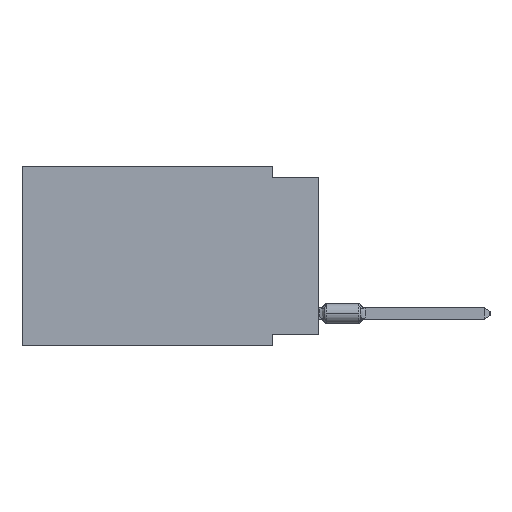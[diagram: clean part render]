
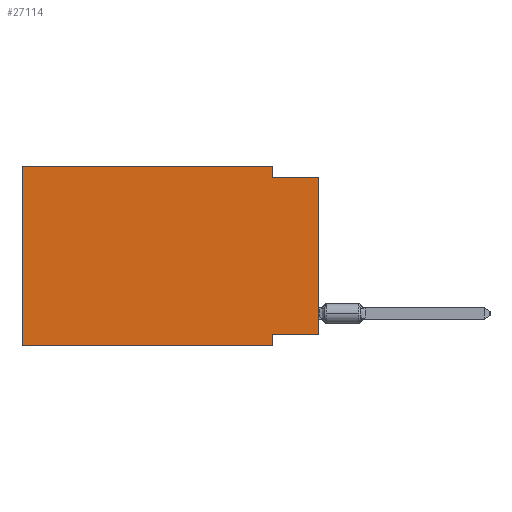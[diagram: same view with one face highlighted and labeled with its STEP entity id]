
A CAD part, left-side view. The second image highlights one B-rep face of the part: STEP entity #27114.
In plain terms, the highlighted planar face has unit normal (-1, 0, 0).
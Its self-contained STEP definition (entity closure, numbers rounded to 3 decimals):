
#895 = DIRECTION ( 'NONE',  ( 0., 0., 1. ) ) ;
#1077 = DIRECTION ( 'NONE',  ( 0., 1., 0. ) ) ;
#1387 = DIRECTION ( 'NONE',  ( 0., 0., -1. ) ) ;
#2608 = VECTOR ( 'NONE', #9329, 1000. ) ;
#2900 = EDGE_CURVE ( 'NONE', #19758, #13571, #29375, .T. ) ;
#4257 = VERTEX_POINT ( 'NONE', #18093 ) ;
#5572 = CARTESIAN_POINT ( 'NONE',  ( 0., 2.54, -9.906 ) ) ;
#6136 = FACE_OUTER_BOUND ( 'NONE', #12895, .T. ) ;
#7039 = EDGE_CURVE ( 'NONE', #14759, #13571, #8423, .T. ) ;
#7259 = ORIENTED_EDGE ( 'NONE', *, *, #7039, .F. ) ;
#8343 = ORIENTED_EDGE ( 'NONE', *, *, #2900, .T. ) ;
#8423 = LINE ( 'NONE', #20137, #11509 ) ;
#8878 = ORIENTED_EDGE ( 'NONE', *, *, #21564, .F. ) ;
#9329 = DIRECTION ( 'NONE',  ( 0., 0., -1. ) ) ;
#9922 = VECTOR ( 'NONE', #16440, 1000. ) ;
#10450 = VECTOR ( 'NONE', #895, 1000. ) ;
#11478 = VERTEX_POINT ( 'NONE', #32034 ) ;
#11509 = VECTOR ( 'NONE', #33464, 1000. ) ;
#12895 = EDGE_LOOP ( 'NONE', ( #8343, #7259, #27799, #15864, #33020, #26986, #20630, #8878 ) ) ;
#13352 = VERTEX_POINT ( 'NONE', #29213 ) ;
#13571 = VERTEX_POINT ( 'NONE', #32173 ) ;
#14233 = LINE ( 'NONE', #27930, #25042 ) ;
#14759 = VERTEX_POINT ( 'NONE', #18105 ) ;
#14871 = LINE ( 'NONE', #30676, #16644 ) ;
#15864 = ORIENTED_EDGE ( 'NONE', *, *, #25416, .F. ) ;
#16440 = DIRECTION ( 'NONE',  ( 0., -1., 0. ) ) ;
#16511 = VECTOR ( 'NONE', #20960, 1000. ) ;
#16644 = VECTOR ( 'NONE', #28745, 1000. ) ;
#18093 = CARTESIAN_POINT ( 'NONE',  ( 0., 16.383, -9.906 ) ) ;
#18105 = CARTESIAN_POINT ( 'NONE',  ( 0., 2.54, -0.635 ) ) ;
#18322 = CARTESIAN_POINT ( 'NONE',  ( 0., 0., 0. ) ) ;
#18431 = VECTOR ( 'NONE', #31993, 1000. ) ;
#19678 = LINE ( 'NONE', #33195, #2608 ) ;
#19758 = VERTEX_POINT ( 'NONE', #32919 ) ;
#20137 = CARTESIAN_POINT ( 'NONE',  ( 0., 0., -0.635 ) ) ;
#20284 = EDGE_CURVE ( 'NONE', #13352, #29763, #14871, .T. ) ;
#20630 = ORIENTED_EDGE ( 'NONE', *, *, #20284, .F. ) ;
#20960 = DIRECTION ( 'NONE',  ( 0., 0., 1. ) ) ;
#21283 = LINE ( 'NONE', #21970, #18431 ) ;
#21564 = EDGE_CURVE ( 'NONE', #19758, #13352, #14233, .T. ) ;
#21599 = EDGE_CURVE ( 'NONE', #27079, #14759, #19678, .T. ) ;
#21616 = EDGE_CURVE ( 'NONE', #4257, #11478, #27582, .T. ) ;
#21970 = CARTESIAN_POINT ( 'NONE',  ( 0., 16.383, 0. ) ) ;
#25042 = VECTOR ( 'NONE', #1077, 1000. ) ;
#25416 = EDGE_CURVE ( 'NONE', #11478, #27079, #21283, .T. ) ;
#26986 = ORIENTED_EDGE ( 'NONE', *, *, #27311, .T. ) ;
#27079 = VERTEX_POINT ( 'NONE', #30191 ) ;
#27114 = ADVANCED_FACE ( 'NONE', ( #6136 ), #30903, .F. ) ;
#27311 = EDGE_CURVE ( 'NONE', #4257, #29763, #34710, .T. ) ;
#27582 = LINE ( 'NONE', #27745, #10450 ) ;
#27745 = CARTESIAN_POINT ( 'NONE',  ( 0., 16.383, 0. ) ) ;
#27799 = ORIENTED_EDGE ( 'NONE', *, *, #21599, .F. ) ;
#27930 = CARTESIAN_POINT ( 'NONE',  ( 0., 0., -9.271 ) ) ;
#28075 = CARTESIAN_POINT ( 'NONE',  ( 0., 16.383, 0. ) ) ;
#28745 = DIRECTION ( 'NONE',  ( 0., 0., -1. ) ) ;
#29213 = CARTESIAN_POINT ( 'NONE',  ( 0., 2.54, -9.271 ) ) ;
#29375 = LINE ( 'NONE', #18322, #16511 ) ;
#29763 = VERTEX_POINT ( 'NONE', #5572 ) ;
#29797 = CARTESIAN_POINT ( 'NONE',  ( 0., 16.383, -9.906 ) ) ;
#30191 = CARTESIAN_POINT ( 'NONE',  ( 0., 2.54, 0. ) ) ;
#30676 = CARTESIAN_POINT ( 'NONE',  ( 0., 2.54, -9.906 ) ) ;
#30903 = PLANE ( 'NONE',  #31989 ) ;
#31989 = AXIS2_PLACEMENT_3D ( 'NONE', #28075, #32811, #1387 ) ;
#31993 = DIRECTION ( 'NONE',  ( 0., -1., 0. ) ) ;
#32034 = CARTESIAN_POINT ( 'NONE',  ( 0., 16.383, 0. ) ) ;
#32173 = CARTESIAN_POINT ( 'NONE',  ( 0., 0., -0.635 ) ) ;
#32811 = DIRECTION ( 'NONE',  ( 1., 0., 0. ) ) ;
#32919 = CARTESIAN_POINT ( 'NONE',  ( 0., 0., -9.271 ) ) ;
#33020 = ORIENTED_EDGE ( 'NONE', *, *, #21616, .F. ) ;
#33195 = CARTESIAN_POINT ( 'NONE',  ( 0., 2.54, 0. ) ) ;
#33464 = DIRECTION ( 'NONE',  ( 0., -1., 0. ) ) ;
#34710 = LINE ( 'NONE', #29797, #9922 ) ;
